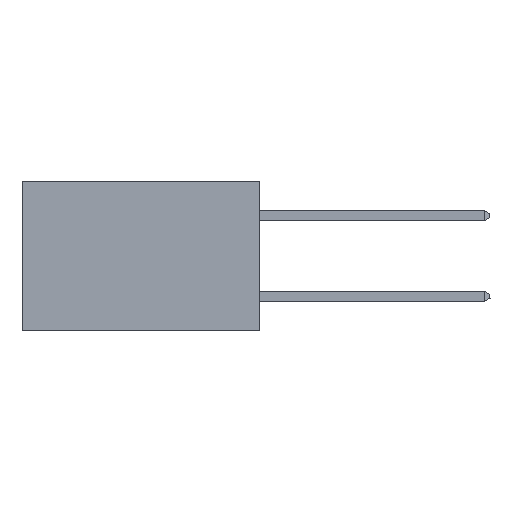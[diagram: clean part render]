
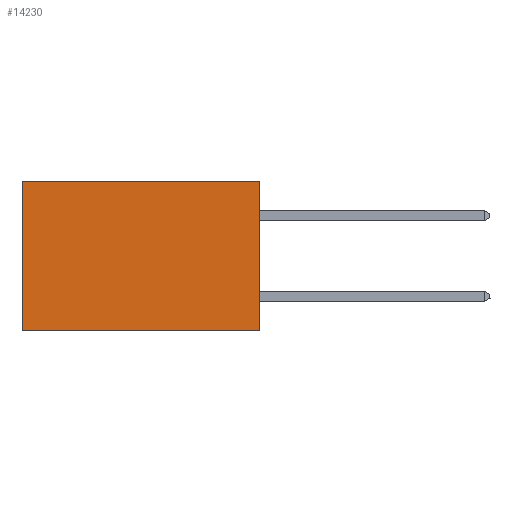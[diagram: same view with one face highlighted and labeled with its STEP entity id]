
A CAD part, left-side view. The second image highlights one B-rep face of the part: STEP entity #14230.
In plain terms, the highlighted planar face has unit normal (-1, 0, 0).
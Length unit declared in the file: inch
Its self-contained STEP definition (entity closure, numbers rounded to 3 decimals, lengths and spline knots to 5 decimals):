
#248 = VECTOR ( 'NONE', #13207, 39.37008 ) ;
#275 = FACE_OUTER_BOUND ( 'NONE', #10630, .T. ) ;
#741 = AXIS2_PLACEMENT_3D ( 'NONE', #15033, #7344, #16325 ) ;
#1565 = VERTEX_POINT ( 'NONE', #10471 ) ;
#2436 = DIRECTION ( 'NONE',  ( 0., 1., 0. ) ) ;
#2814 = LINE ( 'NONE', #11852, #5929 ) ;
#3302 = CARTESIAN_POINT ( 'NONE',  ( 0.277, 0., 0. ) ) ;
#3711 = VERTEX_POINT ( 'NONE', #12740 ) ;
#3772 = LINE ( 'NONE', #8210, #6911 ) ;
#4227 = DIRECTION ( 'NONE',  ( 0., 0., -1. ) ) ;
#4394 = VECTOR ( 'NONE', #2436, 39.37008 ) ;
#4499 = EDGE_CURVE ( 'NONE', #12941, #3711, #2814, .T. ) ;
#5929 = VECTOR ( 'NONE', #11790, 39.37008 ) ;
#6911 = VECTOR ( 'NONE', #4227, 39.37008 ) ;
#7344 = DIRECTION ( 'NONE',  ( 1., 0., 0. ) ) ;
#7736 = ORIENTED_EDGE ( 'NONE', *, *, #16730, .F. ) ;
#8210 = CARTESIAN_POINT ( 'NONE',  ( 0.277, 0.59, -0.37 ) ) ;
#9316 = CARTESIAN_POINT ( 'NONE',  ( 0.277, 0., 0. ) ) ;
#10308 = ORIENTED_EDGE ( 'NONE', *, *, #16141, .T. ) ;
#10471 = CARTESIAN_POINT ( 'NONE',  ( 0.277, 0.59, -0.37 ) ) ;
#10630 = EDGE_LOOP ( 'NONE', ( #14919, #7736, #11468, #10308 ) ) ;
#10751 = EDGE_CURVE ( 'NONE', #16130, #1565, #3772, .T. ) ;
#11468 = ORIENTED_EDGE ( 'NONE', *, *, #4499, .F. ) ;
#11641 = LINE ( 'NONE', #9316, #248 ) ;
#11790 = DIRECTION ( 'NONE',  ( 0., 0., -1. ) ) ;
#11813 = LINE ( 'NONE', #15540, #4394 ) ;
#11852 = CARTESIAN_POINT ( 'NONE',  ( 0.277, 0., -0.37 ) ) ;
#12740 = CARTESIAN_POINT ( 'NONE',  ( 0.277, 0., -0.37 ) ) ;
#12941 = VERTEX_POINT ( 'NONE', #3302 ) ;
#13207 = DIRECTION ( 'NONE',  ( 0., 1., 0. ) ) ;
#13782 = PLANE ( 'NONE',  #741 ) ;
#14230 = ADVANCED_FACE ( 'NONE', ( #275 ), #13782, .F. ) ;
#14400 = CARTESIAN_POINT ( 'NONE',  ( 0.277, 0.59, 0. ) ) ;
#14919 = ORIENTED_EDGE ( 'NONE', *, *, #10751, .T. ) ;
#15033 = CARTESIAN_POINT ( 'NONE',  ( 0.277, 0., -0.37 ) ) ;
#15540 = CARTESIAN_POINT ( 'NONE',  ( 0.277, 0., -0.37 ) ) ;
#16130 = VERTEX_POINT ( 'NONE', #14400 ) ;
#16141 = EDGE_CURVE ( 'NONE', #12941, #16130, #11641, .T. ) ;
#16325 = DIRECTION ( 'NONE',  ( 0., 0., -1. ) ) ;
#16730 = EDGE_CURVE ( 'NONE', #3711, #1565, #11813, .T. ) ;
